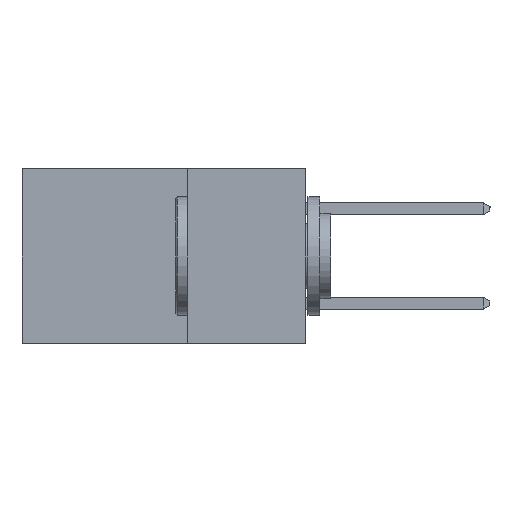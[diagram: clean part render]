
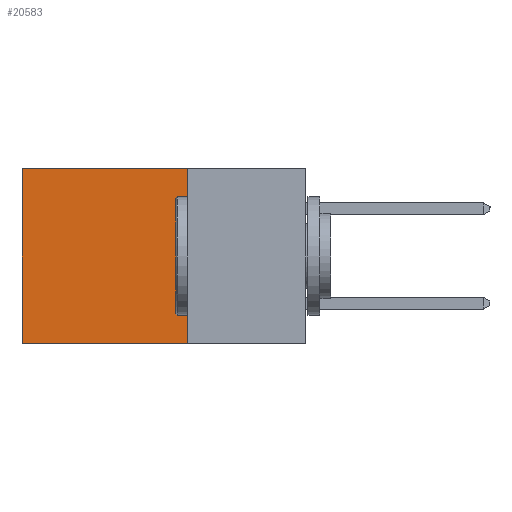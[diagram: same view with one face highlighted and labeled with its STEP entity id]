
A CAD part, left-side view. The second image highlights one B-rep face of the part: STEP entity #20583.
In plain terms, the highlighted planar face has unit normal (-1, 0, 0).
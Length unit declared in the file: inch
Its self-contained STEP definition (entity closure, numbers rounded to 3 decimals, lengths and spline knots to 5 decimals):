
#1389 = VERTEX_POINT ( 'NONE', #5262 ) ;
#1655 = CARTESIAN_POINT ( 'NONE',  ( 0.2615, 0.6, 0. ) ) ;
#2233 = DIRECTION ( 'NONE',  ( 0., 1., 0. ) ) ;
#2845 = CARTESIAN_POINT ( 'NONE',  ( 0.2615, 0.25, -0.37 ) ) ;
#3160 = LINE ( 'NONE', #20485, #20534 ) ;
#5262 = CARTESIAN_POINT ( 'NONE',  ( 0.2615, 0.6, -0.37 ) ) ;
#5710 = EDGE_CURVE ( 'NONE', #8269, #12109, #21600, .T. ) ;
#6228 = VERTEX_POINT ( 'NONE', #24358 ) ;
#7016 = DIRECTION ( 'NONE',  ( 0., 0., -1. ) ) ;
#7309 = DIRECTION ( 'NONE',  ( 0., 1., 0. ) ) ;
#8269 = VERTEX_POINT ( 'NONE', #17203 ) ;
#9465 = LINE ( 'NONE', #11511, #24448 ) ;
#9488 = AXIS2_PLACEMENT_3D ( 'NONE', #2845, #23868, #10617 ) ;
#9622 = EDGE_CURVE ( 'NONE', #8269, #6228, #3160, .T. ) ;
#10617 = DIRECTION ( 'NONE',  ( 0., 0., -1. ) ) ;
#11511 = CARTESIAN_POINT ( 'NONE',  ( 0.2615, 0.25, -0.37 ) ) ;
#12109 = VERTEX_POINT ( 'NONE', #1655 ) ;
#12536 = FACE_OUTER_BOUND ( 'NONE', #22832, .T. ) ;
#13760 = VECTOR ( 'NONE', #2233, 39.37008 ) ;
#13995 = ORIENTED_EDGE ( 'NONE', *, *, #5710, .T. ) ;
#16140 = CARTESIAN_POINT ( 'NONE',  ( 0.2615, 0.25, 0. ) ) ;
#16463 = CARTESIAN_POINT ( 'NONE',  ( 0.2615, 0.6, -0.37 ) ) ;
#16475 = ORIENTED_EDGE ( 'NONE', *, *, #9622, .F. ) ;
#17203 = CARTESIAN_POINT ( 'NONE',  ( 0.2615, 0.25, 0. ) ) ;
#20013 = ORIENTED_EDGE ( 'NONE', *, *, #24173, .F. ) ;
#20306 = PLANE ( 'NONE',  #9488 ) ;
#20485 = CARTESIAN_POINT ( 'NONE',  ( 0.2615, 0.25, -0.37 ) ) ;
#20504 = VECTOR ( 'NONE', #7016, 39.37008 ) ;
#20534 = VECTOR ( 'NONE', #24302, 39.37008 ) ;
#20583 = ADVANCED_FACE ( 'NONE', ( #12536 ), #20306, .F. ) ;
#20653 = LINE ( 'NONE', #16463, #20504 ) ;
#21115 = EDGE_CURVE ( 'NONE', #12109, #1389, #20653, .T. ) ;
#21600 = LINE ( 'NONE', #16140, #13760 ) ;
#22568 = ORIENTED_EDGE ( 'NONE', *, *, #21115, .T. ) ;
#22832 = EDGE_LOOP ( 'NONE', ( #22568, #20013, #16475, #13995 ) ) ;
#23868 = DIRECTION ( 'NONE',  ( 1., 0., 0. ) ) ;
#24173 = EDGE_CURVE ( 'NONE', #6228, #1389, #9465, .T. ) ;
#24302 = DIRECTION ( 'NONE',  ( 0., 0., -1. ) ) ;
#24358 = CARTESIAN_POINT ( 'NONE',  ( 0.2615, 0.25, -0.37 ) ) ;
#24448 = VECTOR ( 'NONE', #7309, 39.37008 ) ;
